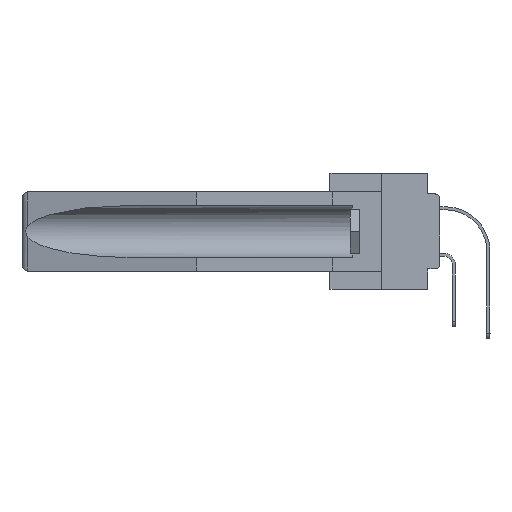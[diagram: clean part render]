
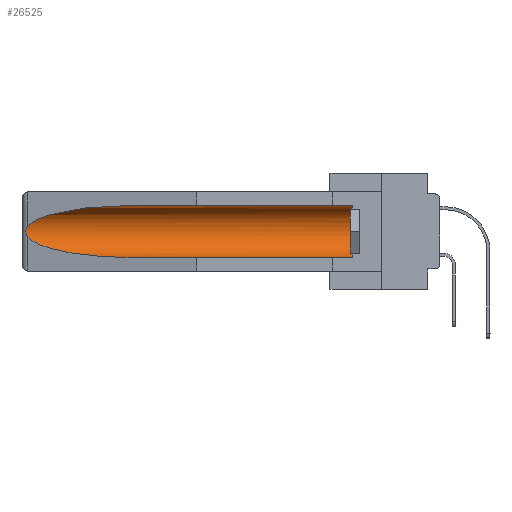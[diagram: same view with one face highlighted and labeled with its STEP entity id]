
A CAD part, left-side view. The second image highlights one B-rep face of the part: STEP entity #26525.
In plain terms, the highlighted cylindrical face has radius 2.857 mm (diameter 5.715 mm), a partial arc.
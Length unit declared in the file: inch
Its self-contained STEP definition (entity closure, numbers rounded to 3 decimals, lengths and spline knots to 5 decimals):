
#50 = CARTESIAN_POINT ( 'NONE',  ( 0.155, 1.07973, -0.284 ) ) ;
#832 = EDGE_CURVE ( 'NONE', #17452, #5668, #9517, .T. ) ;
#1930 = CARTESIAN_POINT ( 'NONE',  ( 0.155, 0.126, -0.284 ) ) ;
#2112 = CARTESIAN_POINT ( 'NONE',  ( 0.155, -0.30754, -0.1715 ) ) ;
#2831 = CARTESIAN_POINT ( 'NONE',  ( 0.155, 1.07973, -0.059 ) ) ;
#4402 = DIRECTION ( 'NONE',  ( 0., 0., 1. ) ) ;
#5496 = CARTESIAN_POINT ( 'NONE',  ( 0.26537, 1.52718, -0.19328 ) ) ;
#5668 = VERTEX_POINT ( 'NONE', #2831 ) ;
#5764 = EDGE_CURVE ( 'NONE', #9948, #13071, #32532, .T. ) ;
#6141 = ORIENTED_EDGE ( 'NONE', *, *, #14785, .F. ) ;
#7062 = VERTEX_POINT ( 'NONE', #1930 ) ;
#8865 = DIRECTION ( 'NONE',  ( 0., 1., 0. ) ) ;
#9254 = EDGE_CURVE ( 'NONE', #5668, #20980, #26007, .T. ) ;
#9337 = CARTESIAN_POINT ( 'NONE',  ( 0.155, -0.30754, -0.059 ) ) ;
#9517 = LINE ( 'NONE', #9337, #22780 ) ;
#9832 = CARTESIAN_POINT ( 'NONE',  ( 0.26537, 1.52718, -0.14972 ) ) ;
#9861 = ORIENTED_EDGE ( 'NONE', *, *, #832, .T. ) ;
#9948 = VERTEX_POINT ( 'NONE', #35439 ) ;
#10014 = CARTESIAN_POINT ( 'NONE',  ( 0.26654, 1.53092, -0.15636 ) ) ;
#11950 = CIRCLE ( 'NONE', #33714, 0.1125 ) ;
#13034 = CARTESIAN_POINT ( 'NONE',  ( 0.25451, 1.48313, -0.09465 ) ) ;
#13071 = VERTEX_POINT ( 'NONE', #50 ) ;
#14785 = EDGE_CURVE ( 'NONE', #7062, #13071, #17395, .T. ) ;
#15468 = B_SPLINE_CURVE_WITH_KNOTS ( 'NONE', 3,
 ( #9832, #35807, #10014, #30672, #21212, #27064, #21393, #32959, #32780, #30480 ),
 .UNSPECIFIED., .F., .F.,
 ( 4, 2, 2, 2, 4 ),
 ( 0., 0.00029, 0.00058, 0.00087, 0.00117 ),
 .UNSPECIFIED. ) ;
#15574 = EDGE_CURVE ( 'NONE', #20980, #9948, #15468, .T. ) ;
#15950 = ORIENTED_EDGE ( 'NONE', *, *, #15574, .T. ) ;
#17395 = LINE ( 'NONE', #34642, #37241 ) ;
#17452 = VERTEX_POINT ( 'NONE', #27404 ) ;
#18812 = DIRECTION ( 'NONE',  ( 0., -1., 0. ) ) ;
#18911 = CARTESIAN_POINT ( 'NONE',  ( 0.155, 1.07973, -0.059 ) ) ;
#18994 = DIRECTION ( 'NONE',  ( 0., 0., 1. ) ) ;
#20091 = CARTESIAN_POINT ( 'NONE',  ( 0.21114, 1.30732, -0.284 ) ) ;
#20980 = VERTEX_POINT ( 'NONE', #29682 ) ;
#21075 = DIRECTION ( 'NONE',  ( 0., 1., 0. ) ) ;
#21181 = CARTESIAN_POINT ( 'NONE',  ( 0.26537, 1.52718, -0.14972 ) ) ;
#21212 = CARTESIAN_POINT ( 'NONE',  ( 0.2675, 1.53308, -0.16763 ) ) ;
#21393 = CARTESIAN_POINT ( 'NONE',  ( 0.2673, 1.53269, -0.17917 ) ) ;
#22780 = VECTOR ( 'NONE', #21075, 39.37008 ) ;
#23580 = EDGE_LOOP ( 'NONE', ( #32739, #15950, #25912, #6141, #35455, #9861 ) ) ;
#24024 = CARTESIAN_POINT ( 'NONE',  ( 0.155, 1.07973, -0.284 ) ) ;
#25912 = ORIENTED_EDGE ( 'NONE', *, *, #5764, .T. ) ;
#26007 =( BOUNDED_CURVE ( )  B_SPLINE_CURVE ( 3, ( #18911, #35398, #13034, #21181 ),
 .UNSPECIFIED., .F., .T. ) 
 B_SPLINE_CURVE_WITH_KNOTS ( ( 4, 4 ),
 ( 4.71239, 6.08839 ),
 .UNSPECIFIED. ) 
 CURVE ( )  GEOMETRIC_REPRESENTATION_ITEM ( )  RATIONAL_B_SPLINE_CURVE ( ( 1., 0.848, 0.848, 1. ) ) 
 REPRESENTATION_ITEM ( '' )  );
#26486 = EDGE_CURVE ( 'NONE', #7062, #17452, #11950, .T. ) ;
#26525 = ADVANCED_FACE ( 'NONE', ( #36242 ), #33396, .F. ) ;
#27064 = CARTESIAN_POINT ( 'NONE',  ( 0.2675, 1.53308, -0.17534 ) ) ;
#27404 = CARTESIAN_POINT ( 'NONE',  ( 0.155, 0.126, -0.059 ) ) ;
#28049 = CARTESIAN_POINT ( 'NONE',  ( 0.155, 0.126, -0.1715 ) ) ;
#29682 = CARTESIAN_POINT ( 'NONE',  ( 0.26537, 1.52718, -0.14972 ) ) ;
#30480 = CARTESIAN_POINT ( 'NONE',  ( 0.26537, 1.52718, -0.19328 ) ) ;
#30672 = CARTESIAN_POINT ( 'NONE',  ( 0.2673, 1.5327, -0.16383 ) ) ;
#32532 =( BOUNDED_CURVE ( )  B_SPLINE_CURVE ( 3, ( #5496, #34485, #20091, #24024 ),
 .UNSPECIFIED., .F., .T. ) 
 B_SPLINE_CURVE_WITH_KNOTS ( ( 4, 4 ),
 ( 0.1948, 1.5708 ),
 .UNSPECIFIED. ) 
 CURVE ( )  GEOMETRIC_REPRESENTATION_ITEM ( )  RATIONAL_B_SPLINE_CURVE ( ( 1., 0.848, 0.848, 1. ) ) 
 REPRESENTATION_ITEM ( '' )  );
#32739 = ORIENTED_EDGE ( 'NONE', *, *, #9254, .T. ) ;
#32780 = CARTESIAN_POINT ( 'NONE',  ( 0.26597, 1.5296, -0.19026 ) ) ;
#32959 = CARTESIAN_POINT ( 'NONE',  ( 0.26655, 1.53094, -0.18657 ) ) ;
#33122 = AXIS2_PLACEMENT_3D ( 'NONE', #2112, #33572, #18994 ) ;
#33396 = CYLINDRICAL_SURFACE ( 'NONE', #33122, 0.1125 ) ;
#33572 = DIRECTION ( 'NONE',  ( 0., 1., 0. ) ) ;
#33714 = AXIS2_PLACEMENT_3D ( 'NONE', #28049, #18812, #4402 ) ;
#34485 = CARTESIAN_POINT ( 'NONE',  ( 0.25451, 1.48313, -0.24835 ) ) ;
#34642 = CARTESIAN_POINT ( 'NONE',  ( 0.155, -0.30754, -0.284 ) ) ;
#35398 = CARTESIAN_POINT ( 'NONE',  ( 0.21114, 1.30732, -0.059 ) ) ;
#35439 = CARTESIAN_POINT ( 'NONE',  ( 0.26537, 1.52718, -0.19328 ) ) ;
#35455 = ORIENTED_EDGE ( 'NONE', *, *, #26486, .T. ) ;
#35807 = CARTESIAN_POINT ( 'NONE',  ( 0.26597, 1.52961, -0.15275 ) ) ;
#36242 = FACE_OUTER_BOUND ( 'NONE', #23580, .T. ) ;
#37241 = VECTOR ( 'NONE', #8865, 39.37008 ) ;
